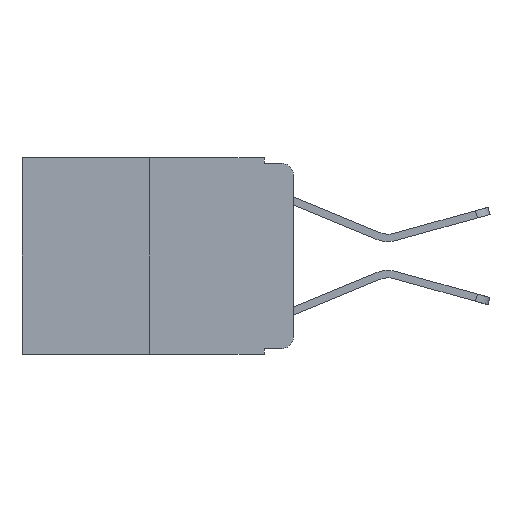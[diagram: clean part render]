
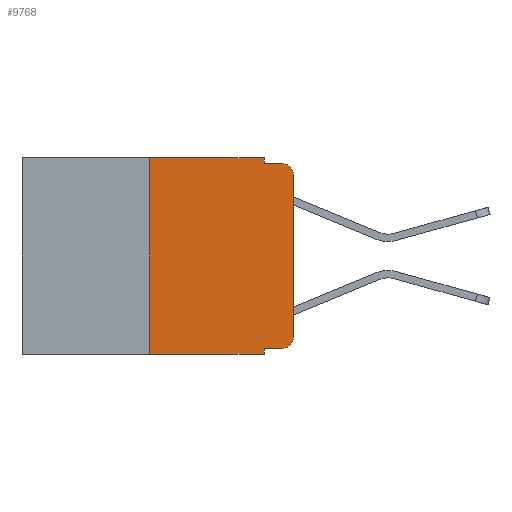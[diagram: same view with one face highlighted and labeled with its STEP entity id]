
A CAD part, left-side view. The second image highlights one B-rep face of the part: STEP entity #9768.
In plain terms, the highlighted planar face has unit normal (-1, 0, 0).
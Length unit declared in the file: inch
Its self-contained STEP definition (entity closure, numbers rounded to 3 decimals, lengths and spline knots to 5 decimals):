
#101 = VERTEX_POINT ( 'NONE', #18489 ) ;
#321 = CARTESIAN_POINT ( 'NONE',  ( 0., 0.051, -0.343 ) ) ;
#1316 = ORIENTED_EDGE ( 'NONE', *, *, #7005, .F. ) ;
#1409 = CARTESIAN_POINT ( 'NONE',  ( 0., 0.473, -0.343 ) ) ;
#1420 = LINE ( 'NONE', #19711, #18245 ) ;
#1435 = CARTESIAN_POINT ( 'NONE',  ( 0., 0.25, -0.343 ) ) ;
#1536 = DIRECTION ( 'NONE',  ( 0., 0., -1. ) ) ;
#1575 = ORIENTED_EDGE ( 'NONE', *, *, #18033, .T. ) ;
#1663 = VERTEX_POINT ( 'NONE', #14787 ) ;
#1753 = LINE ( 'NONE', #1409, #19098 ) ;
#2088 = CARTESIAN_POINT ( 'NONE',  ( 0., 0.473, 0. ) ) ;
#2920 = CARTESIAN_POINT ( 'NONE',  ( 0., 0.051, -0.01 ) ) ;
#3229 = ORIENTED_EDGE ( 'NONE', *, *, #5757, .T. ) ;
#3238 = LINE ( 'NONE', #11718, #11707 ) ;
#3366 = CARTESIAN_POINT ( 'NONE',  ( 0., 0.02, -0.333 ) ) ;
#3379 = EDGE_CURVE ( 'NONE', #101, #11716, #14029, .T. ) ;
#3737 = ORIENTED_EDGE ( 'NONE', *, *, #3379, .T. ) ;
#3837 = DIRECTION ( 'NONE',  ( 0., 0., -1. ) ) ;
#3876 = EDGE_CURVE ( 'NONE', #4955, #18392, #20212, .T. ) ;
#3987 = CARTESIAN_POINT ( 'NONE',  ( 0., 0.02, -0.03 ) ) ;
#4673 = DIRECTION ( 'NONE',  ( 0., 0., 1. ) ) ;
#4955 = VERTEX_POINT ( 'NONE', #9646 ) ;
#5089 = ORIENTED_EDGE ( 'NONE', *, *, #5808, .T. ) ;
#5110 = VERTEX_POINT ( 'NONE', #1435 ) ;
#5718 = DIRECTION ( 'NONE',  ( 0., 0., -1. ) ) ;
#5757 = EDGE_CURVE ( 'NONE', #6735, #101, #11365, .T. ) ;
#5808 = EDGE_CURVE ( 'NONE', #5110, #18392, #1753, .T. ) ;
#6187 = EDGE_CURVE ( 'NONE', #19317, #1663, #7977, .T. ) ;
#6720 = FACE_OUTER_BOUND ( 'NONE', #9041, .T. ) ;
#6735 = VERTEX_POINT ( 'NONE', #3366 ) ;
#7005 = EDGE_CURVE ( 'NONE', #21459, #18158, #7402, .T. ) ;
#7402 = LINE ( 'NONE', #14437, #15661 ) ;
#7779 = EDGE_CURVE ( 'NONE', #5110, #19317, #1420, .T. ) ;
#7977 = LINE ( 'NONE', #19378, #20115 ) ;
#8326 = ORIENTED_EDGE ( 'NONE', *, *, #11619, .T. ) ;
#8429 = DIRECTION ( 'NONE',  ( -1., 0., 0. ) ) ;
#9041 = EDGE_LOOP ( 'NONE', ( #3737, #8326, #1316, #19700, #20201, #12970, #5089, #14507, #1575, #3229 ) ) ;
#9169 = VECTOR ( 'NONE', #17503, 39.37008 ) ;
#9646 = CARTESIAN_POINT ( 'NONE',  ( 0., 0.051, -0.333 ) ) ;
#9768 = ADVANCED_FACE ( 'NONE', ( #6720 ), #10595, .F. ) ;
#10021 = CARTESIAN_POINT ( 'NONE',  ( 0., 0.051, 0. ) ) ;
#10162 = DIRECTION ( 'NONE',  ( 0., -1., 0. ) ) ;
#10183 = AXIS2_PLACEMENT_3D ( 'NONE', #2088, #13891, #3837 ) ;
#10595 = PLANE ( 'NONE',  #10183 ) ;
#11151 = DIRECTION ( 'NONE',  ( 0., -1., 0. ) ) ;
#11331 = VECTOR ( 'NONE', #17862, 39.37008 ) ;
#11365 = CIRCLE ( 'NONE', #15736, 0.02 ) ;
#11619 = EDGE_CURVE ( 'NONE', #11716, #18158, #18846, .T. ) ;
#11707 = VECTOR ( 'NONE', #1536, 39.37008 ) ;
#11716 = VERTEX_POINT ( 'NONE', #15894 ) ;
#11718 = CARTESIAN_POINT ( 'NONE',  ( 0., 0.051, 0. ) ) ;
#12970 = ORIENTED_EDGE ( 'NONE', *, *, #7779, .F. ) ;
#13664 = CARTESIAN_POINT ( 'NONE',  ( 0., 0., 0. ) ) ;
#13891 = DIRECTION ( 'NONE',  ( 1., 0., 0. ) ) ;
#14029 = LINE ( 'NONE', #13664, #9169 ) ;
#14437 = CARTESIAN_POINT ( 'NONE',  ( 0., 0.051, -0.01 ) ) ;
#14507 = ORIENTED_EDGE ( 'NONE', *, *, #3876, .F. ) ;
#14787 = CARTESIAN_POINT ( 'NONE',  ( 0., 0.051, 0. ) ) ;
#15661 = VECTOR ( 'NONE', #19463, 39.37008 ) ;
#15682 = DIRECTION ( 'NONE',  ( -1., 0., 0. ) ) ;
#15683 = LINE ( 'NONE', #16171, #11331 ) ;
#15736 = AXIS2_PLACEMENT_3D ( 'NONE', #18305, #8429, #19961 ) ;
#15793 = VECTOR ( 'NONE', #21491, 39.37008 ) ;
#15894 = CARTESIAN_POINT ( 'NONE',  ( 0., 0., -0.03 ) ) ;
#16171 = CARTESIAN_POINT ( 'NONE',  ( 0., 0.051, -0.333 ) ) ;
#16464 = CARTESIAN_POINT ( 'NONE',  ( 0., 0.02, -0.01 ) ) ;
#16551 = AXIS2_PLACEMENT_3D ( 'NONE', #3987, #15682, #5718 ) ;
#17503 = DIRECTION ( 'NONE',  ( 0., 0., 1. ) ) ;
#17862 = DIRECTION ( 'NONE',  ( 0., -1., 0. ) ) ;
#18033 = EDGE_CURVE ( 'NONE', #4955, #6735, #15683, .T. ) ;
#18158 = VERTEX_POINT ( 'NONE', #16464 ) ;
#18245 = VECTOR ( 'NONE', #4673, 39.37008 ) ;
#18305 = CARTESIAN_POINT ( 'NONE',  ( 0., 0.02, -0.313 ) ) ;
#18392 = VERTEX_POINT ( 'NONE', #321 ) ;
#18489 = CARTESIAN_POINT ( 'NONE',  ( 0., 0., -0.313 ) ) ;
#18846 = CIRCLE ( 'NONE', #16551, 0.02 ) ;
#19098 = VECTOR ( 'NONE', #10162, 39.37008 ) ;
#19317 = VERTEX_POINT ( 'NONE', #21242 ) ;
#19378 = CARTESIAN_POINT ( 'NONE',  ( 0., 0.473, 0. ) ) ;
#19463 = DIRECTION ( 'NONE',  ( 0., -1., 0. ) ) ;
#19700 = ORIENTED_EDGE ( 'NONE', *, *, #21546, .F. ) ;
#19711 = CARTESIAN_POINT ( 'NONE',  ( 0., 0.25, 0. ) ) ;
#19961 = DIRECTION ( 'NONE',  ( 0., 0., -1. ) ) ;
#20115 = VECTOR ( 'NONE', #11151, 39.37008 ) ;
#20201 = ORIENTED_EDGE ( 'NONE', *, *, #6187, .F. ) ;
#20212 = LINE ( 'NONE', #10021, #15793 ) ;
#21242 = CARTESIAN_POINT ( 'NONE',  ( 0., 0.25, 0. ) ) ;
#21459 = VERTEX_POINT ( 'NONE', #2920 ) ;
#21491 = DIRECTION ( 'NONE',  ( 0., 0., -1. ) ) ;
#21546 = EDGE_CURVE ( 'NONE', #1663, #21459, #3238, .T. ) ;
